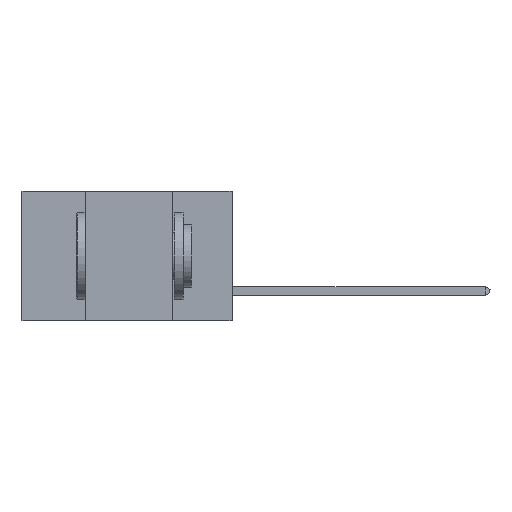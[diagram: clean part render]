
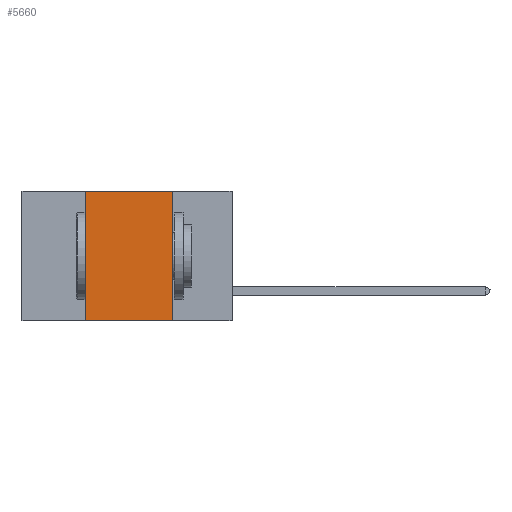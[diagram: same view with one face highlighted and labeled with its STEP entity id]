
A CAD part, left-side view. The second image highlights one B-rep face of the part: STEP entity #5660.
In plain terms, the highlighted planar face has unit normal (-1, 0, 0).
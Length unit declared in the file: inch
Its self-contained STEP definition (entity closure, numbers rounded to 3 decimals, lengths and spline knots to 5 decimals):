
#349 = VERTEX_POINT ( 'NONE', #17673 ) ;
#1222 = VECTOR ( 'NONE', #4421, 39.37008 ) ;
#2371 = CARTESIAN_POINT ( 'NONE',  ( 0., 0.17, 0. ) ) ;
#3601 = AXIS2_PLACEMENT_3D ( 'NONE', #8776, #26148, #25648 ) ;
#4421 = DIRECTION ( 'NONE',  ( 0., 0., 1. ) ) ;
#4648 = VERTEX_POINT ( 'NONE', #29282 ) ;
#4668 = ORIENTED_EDGE ( 'NONE', *, *, #27604, .T. ) ;
#5660 = ADVANCED_FACE ( 'NONE', ( #8856 ), #19727, .F. ) ;
#8776 = CARTESIAN_POINT ( 'NONE',  ( 0., 0.6, 0. ) ) ;
#8856 = FACE_OUTER_BOUND ( 'NONE', #19733, .T. ) ;
#8919 = VECTOR ( 'NONE', #25361, 39.37008 ) ;
#9007 = LINE ( 'NONE', #9051, #1222 ) ;
#9051 = CARTESIAN_POINT ( 'NONE',  ( 0., 0.42, 0. ) ) ;
#10010 = EDGE_CURVE ( 'NONE', #4648, #16795, #9007, .T. ) ;
#10173 = EDGE_CURVE ( 'NONE', #30754, #349, #27202, .T. ) ;
#10314 = CARTESIAN_POINT ( 'NONE',  ( 0., 0.6, -0.37 ) ) ;
#10660 = DIRECTION ( 'NONE',  ( 0., 0., -1. ) ) ;
#12185 = CARTESIAN_POINT ( 'NONE',  ( 0., 0.17, 0. ) ) ;
#16455 = CARTESIAN_POINT ( 'NONE',  ( 0., 0.42, 0. ) ) ;
#16795 = VERTEX_POINT ( 'NONE', #16455 ) ;
#17673 = CARTESIAN_POINT ( 'NONE',  ( 0., 0.17, -0.37 ) ) ;
#19727 = PLANE ( 'NONE',  #3601 ) ;
#19733 = EDGE_LOOP ( 'NONE', ( #26244, #22841, #32801, #4668 ) ) ;
#22841 = ORIENTED_EDGE ( 'NONE', *, *, #32980, .F. ) ;
#24401 = LINE ( 'NONE', #10314, #8919 ) ;
#24990 = DIRECTION ( 'NONE',  ( 0., -1., 0. ) ) ;
#25361 = DIRECTION ( 'NONE',  ( 0., -1., 0. ) ) ;
#25648 = DIRECTION ( 'NONE',  ( 0., 0., -1. ) ) ;
#26148 = DIRECTION ( 'NONE',  ( 1., 0., 0. ) ) ;
#26244 = ORIENTED_EDGE ( 'NONE', *, *, #10173, .F. ) ;
#27202 = LINE ( 'NONE', #2371, #37217 ) ;
#27604 = EDGE_CURVE ( 'NONE', #4648, #349, #24401, .T. ) ;
#29231 = VECTOR ( 'NONE', #24990, 39.37008 ) ;
#29282 = CARTESIAN_POINT ( 'NONE',  ( 0., 0.42, -0.37 ) ) ;
#30098 = CARTESIAN_POINT ( 'NONE',  ( 0., 0.6, 0. ) ) ;
#30754 = VERTEX_POINT ( 'NONE', #12185 ) ;
#32801 = ORIENTED_EDGE ( 'NONE', *, *, #10010, .F. ) ;
#32980 = EDGE_CURVE ( 'NONE', #16795, #30754, #37405, .T. ) ;
#37217 = VECTOR ( 'NONE', #10660, 39.37008 ) ;
#37405 = LINE ( 'NONE', #30098, #29231 ) ;
